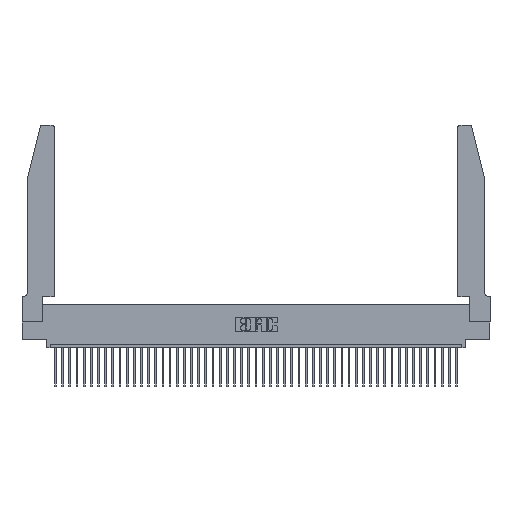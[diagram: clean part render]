
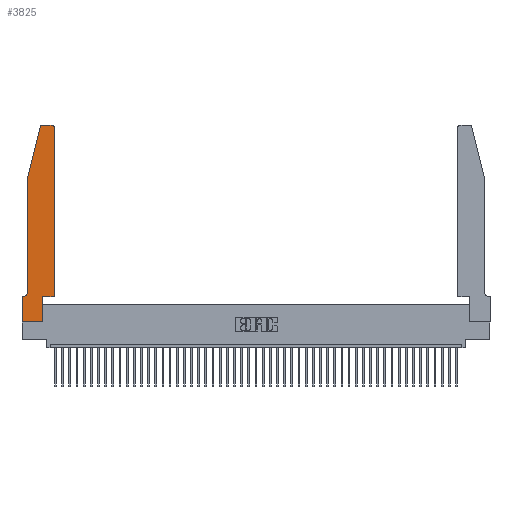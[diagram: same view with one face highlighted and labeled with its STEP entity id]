
A CAD part, top view. The second image highlights one B-rep face of the part: STEP entity #3825.
In plain terms, the highlighted planar face has unit normal (0, 0, 1).
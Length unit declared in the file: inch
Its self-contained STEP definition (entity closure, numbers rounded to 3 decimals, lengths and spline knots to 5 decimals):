
#105 = ORIENTED_EDGE ( 'NONE', *, *, #30289, .T. ) ;
#415 = EDGE_CURVE ( 'NONE', #6517, #13505, #19234, .T. ) ;
#1193 = AXIS2_PLACEMENT_3D ( 'NONE', #25110, #3916, #7920 ) ;
#1777 = EDGE_CURVE ( 'NONE', #43121, #3523, #24714, .T. ) ;
#1835 = VECTOR ( 'NONE', #14949, 39.37008 ) ;
#2145 = EDGE_CURVE ( 'NONE', #15357, #5058, #30207, .T. ) ;
#2672 = DIRECTION ( 'NONE',  ( 0., 0., -1. ) ) ;
#2688 = VECTOR ( 'NONE', #27074, 39.37008 ) ;
#2939 = VERTEX_POINT ( 'NONE', #25830 ) ;
#3291 = FACE_OUTER_BOUND ( 'NONE', #38762, .T. ) ;
#3523 = VERTEX_POINT ( 'NONE', #16268 ) ;
#3825 = ADVANCED_FACE ( 'NONE', ( #3291 ), #8225, .T. ) ;
#3916 = DIRECTION ( 'NONE',  ( 0., 0., 1. ) ) ;
#4210 = VERTEX_POINT ( 'NONE', #18796 ) ;
#5058 = VERTEX_POINT ( 'NONE', #21980 ) ;
#6021 = CARTESIAN_POINT ( 'NONE',  ( 0.0055, 0.35, 0.37 ) ) ;
#6124 = ORIENTED_EDGE ( 'NONE', *, *, #44425, .T. ) ;
#6249 = EDGE_CURVE ( 'NONE', #4210, #22553, #42804, .T. ) ;
#6517 = VERTEX_POINT ( 'NONE', #41214 ) ;
#6872 = CARTESIAN_POINT ( 'NONE',  ( 0.4505, 0.35, 0.37 ) ) ;
#6936 = VECTOR ( 'NONE', #45238, 39.37008 ) ;
#7008 = CIRCLE ( 'NONE', #28515, 0.03 ) ;
#7746 = CARTESIAN_POINT ( 'NONE',  ( 0.2865, 0., 0.37 ) ) ;
#7920 = DIRECTION ( 'NONE',  ( 1., 0., 0. ) ) ;
#8225 = PLANE ( 'NONE',  #40344 ) ;
#9237 = ORIENTED_EDGE ( 'NONE', *, *, #35618, .T. ) ;
#9967 = VERTEX_POINT ( 'NONE', #44963 ) ;
#9983 = CARTESIAN_POINT ( 'NONE',  ( 0.4505, 2.72, 0.37 ) ) ;
#10137 = DIRECTION ( 'NONE',  ( -1., 0., 0. ) ) ;
#11317 = EDGE_CURVE ( 'NONE', #2939, #4210, #7008, .T. ) ;
#12485 = ORIENTED_EDGE ( 'NONE', *, *, #44290, .T. ) ;
#13374 = CARTESIAN_POINT ( 'NONE',  ( 0., 0., 0.37 ) ) ;
#13505 = VERTEX_POINT ( 'NONE', #13374 ) ;
#14193 = VECTOR ( 'NONE', #43222, 39.37008 ) ;
#14949 = DIRECTION ( 'NONE',  ( -1., 0., 0. ) ) ;
#15327 = AXIS2_PLACEMENT_3D ( 'NONE', #42111, #2672, #41795 ) ;
#15347 = DIRECTION ( 'NONE',  ( 1., 0., 0. ) ) ;
#15357 = VERTEX_POINT ( 'NONE', #9983 ) ;
#15961 = DIRECTION ( 'NONE',  ( 0., 0., 1. ) ) ;
#16268 = CARTESIAN_POINT ( 'NONE',  ( 0.2865, 0.35, 0.37 ) ) ;
#16752 = CARTESIAN_POINT ( 'NONE',  ( 0.0755, 2., 0.37 ) ) ;
#18682 = ORIENTED_EDGE ( 'NONE', *, *, #6249, .T. ) ;
#18796 = CARTESIAN_POINT ( 'NONE',  ( 0.25487, 2.72718, 0.37 ) ) ;
#19234 = LINE ( 'NONE', #27243, #2688 ) ;
#19293 = ORIENTED_EDGE ( 'NONE', *, *, #19950, .T. ) ;
#19328 = LINE ( 'NONE', #23330, #25403 ) ;
#19377 = CARTESIAN_POINT ( 'NONE',  ( 0.284, 2.72, 0.37 ) ) ;
#19393 = VECTOR ( 'NONE', #10137, 39.37008 ) ;
#19950 = EDGE_CURVE ( 'NONE', #29142, #15357, #41908, .T. ) ;
#20013 = DIRECTION ( 'NONE',  ( 0., 1., 0. ) ) ;
#20404 = VECTOR ( 'NONE', #35181, 39.37008 ) ;
#20475 = ORIENTED_EDGE ( 'NONE', *, *, #11317, .T. ) ;
#20525 = CARTESIAN_POINT ( 'NONE',  ( 0., 0., 0.37 ) ) ;
#21980 = CARTESIAN_POINT ( 'NONE',  ( 0.4205, 2.75, 0.37 ) ) ;
#22553 = VERTEX_POINT ( 'NONE', #39024 ) ;
#23097 = CARTESIAN_POINT ( 'NONE',  ( 0., 0.35, 0.37 ) ) ;
#23330 = CARTESIAN_POINT ( 'NONE',  ( 0.0755, 2., 0.37 ) ) ;
#23359 = LINE ( 'NONE', #37959, #19393 ) ;
#23480 = DIRECTION ( 'NONE',  ( 0., -1., 0. ) ) ;
#24714 = LINE ( 'NONE', #26516, #37995 ) ;
#25110 = CARTESIAN_POINT ( 'NONE',  ( 0.4205, 2.72, 0.37 ) ) ;
#25254 = DIRECTION ( 'NONE',  ( 1., 0., 0. ) ) ;
#25403 = VECTOR ( 'NONE', #23480, 39.37008 ) ;
#25830 = CARTESIAN_POINT ( 'NONE',  ( 0.284, 2.75, 0.37 ) ) ;
#26122 = CARTESIAN_POINT ( 'NONE',  ( 0.2605, 2.75, 0.37 ) ) ;
#26516 = CARTESIAN_POINT ( 'NONE',  ( 0.2865, 0.35, 0.37 ) ) ;
#26824 = ORIENTED_EDGE ( 'NONE', *, *, #415, .T. ) ;
#27074 = DIRECTION ( 'NONE',  ( 0., -1., 0. ) ) ;
#27243 = CARTESIAN_POINT ( 'NONE',  ( 0., 0., 0.37 ) ) ;
#27337 = LINE ( 'NONE', #26122, #1835 ) ;
#27666 = ORIENTED_EDGE ( 'NONE', *, *, #1777, .T. ) ;
#27758 = EDGE_CURVE ( 'NONE', #13505, #43121, #29178, .T. ) ;
#28515 = AXIS2_PLACEMENT_3D ( 'NONE', #19377, #15961, #15347 ) ;
#29142 = VERTEX_POINT ( 'NONE', #41061 ) ;
#29178 = LINE ( 'NONE', #20525, #36981 ) ;
#30207 = CIRCLE ( 'NONE', #1193, 0.03 ) ;
#30289 = EDGE_CURVE ( 'NONE', #5058, #2939, #27337, .T. ) ;
#30720 = ORIENTED_EDGE ( 'NONE', *, *, #2145, .T. ) ;
#31724 = ORIENTED_EDGE ( 'NONE', *, *, #36426, .T. ) ;
#33967 = DIRECTION ( 'NONE',  ( 0., 0., 1. ) ) ;
#35181 = DIRECTION ( 'NONE',  ( 1., 0., 0. ) ) ;
#35527 = VERTEX_POINT ( 'NONE', #6021 ) ;
#35618 = EDGE_CURVE ( 'NONE', #22553, #9967, #19328, .T. ) ;
#36426 = EDGE_CURVE ( 'NONE', #3523, #29142, #39189, .T. ) ;
#36981 = VECTOR ( 'NONE', #25254, 39.37008 ) ;
#37959 = CARTESIAN_POINT ( 'NONE',  ( 0.0755, 0.35, 0.37 ) ) ;
#37995 = VECTOR ( 'NONE', #20013, 39.37008 ) ;
#38333 = CIRCLE ( 'NONE', #15327, 0.07 ) ;
#38762 = EDGE_LOOP ( 'NONE', ( #105, #20475, #18682, #9237, #12485, #6124, #26824, #39491, #27666, #31724, #19293, #30720 ) ) ;
#39024 = CARTESIAN_POINT ( 'NONE',  ( 0.0755, 2., 0.37 ) ) ;
#39189 = LINE ( 'NONE', #6872, #20404 ) ;
#39491 = ORIENTED_EDGE ( 'NONE', *, *, #27758, .T. ) ;
#40344 = AXIS2_PLACEMENT_3D ( 'NONE', #23097, #33967, #44110 ) ;
#41061 = CARTESIAN_POINT ( 'NONE',  ( 0.4505, 0.35, 0.37 ) ) ;
#41214 = CARTESIAN_POINT ( 'NONE',  ( 0., 0.35, 0.37 ) ) ;
#41256 = CARTESIAN_POINT ( 'NONE',  ( 0.4505, 0.35, 0.37 ) ) ;
#41795 = DIRECTION ( 'NONE',  ( -1., 0., 0. ) ) ;
#41908 = LINE ( 'NONE', #41256, #14193 ) ;
#42111 = CARTESIAN_POINT ( 'NONE',  ( 0.0055, 0.42, 0.37 ) ) ;
#42804 = LINE ( 'NONE', #16752, #6936 ) ;
#43121 = VERTEX_POINT ( 'NONE', #7746 ) ;
#43222 = DIRECTION ( 'NONE',  ( 0., 1., 0. ) ) ;
#44110 = DIRECTION ( 'NONE',  ( 1., 0., 0. ) ) ;
#44290 = EDGE_CURVE ( 'NONE', #9967, #35527, #38333, .T. ) ;
#44425 = EDGE_CURVE ( 'NONE', #35527, #6517, #23359, .T. ) ;
#44963 = CARTESIAN_POINT ( 'NONE',  ( 0.0755, 0.42, 0.37 ) ) ;
#45238 = DIRECTION ( 'NONE',  ( -0.239, -0.971, 0. ) ) ;
